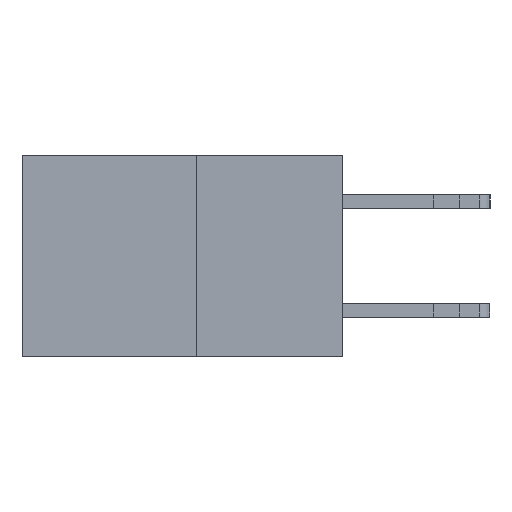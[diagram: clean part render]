
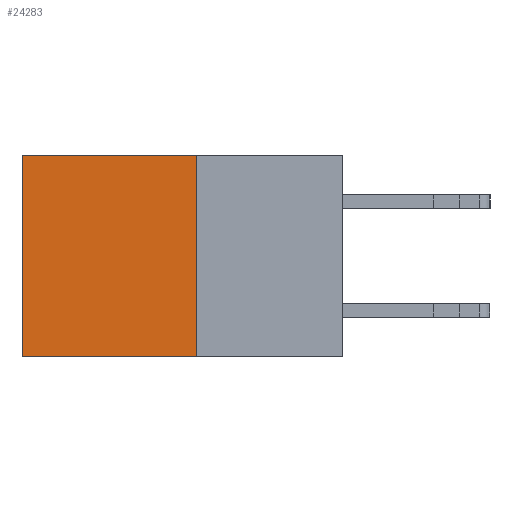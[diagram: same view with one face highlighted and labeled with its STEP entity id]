
A CAD part, left-side view. The second image highlights one B-rep face of the part: STEP entity #24283.
In plain terms, the highlighted planar face has unit normal (-1, 0, 0).
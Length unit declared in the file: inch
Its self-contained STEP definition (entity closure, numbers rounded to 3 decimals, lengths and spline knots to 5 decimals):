
#56 = DIRECTION ( 'NONE',  ( 0., 1., 0. ) ) ;
#512 = LINE ( 'NONE', #28628, #13226 ) ;
#710 = DIRECTION ( 'NONE',  ( 1., 0., 0. ) ) ;
#1823 = CARTESIAN_POINT ( 'NONE',  ( 0.277, 0.27, 0. ) ) ;
#1856 = EDGE_CURVE ( 'NONE', #9199, #30092, #512, .T. ) ;
#2623 = VECTOR ( 'NONE', #16807, 39.37008 ) ;
#3035 = CARTESIAN_POINT ( 'NONE',  ( 0.277, 0.27, -0.37 ) ) ;
#5921 = EDGE_LOOP ( 'NONE', ( #16768, #11929, #25193, #25922 ) ) ;
#8485 = VECTOR ( 'NONE', #22010, 39.37008 ) ;
#9199 = VERTEX_POINT ( 'NONE', #21758 ) ;
#9420 = VERTEX_POINT ( 'NONE', #27135 ) ;
#11929 = ORIENTED_EDGE ( 'NONE', *, *, #1856, .F. ) ;
#12901 = CARTESIAN_POINT ( 'NONE',  ( 0.277, 0.27, 0. ) ) ;
#13226 = VECTOR ( 'NONE', #56, 39.37008 ) ;
#14421 = CARTESIAN_POINT ( 'NONE',  ( 0.277, 0.59, -0.37 ) ) ;
#14996 = PLANE ( 'NONE',  #27520 ) ;
#15300 = EDGE_CURVE ( 'NONE', #21005, #9199, #18866, .T. ) ;
#16246 = FACE_OUTER_BOUND ( 'NONE', #5921, .T. ) ;
#16768 = ORIENTED_EDGE ( 'NONE', *, *, #21220, .T. ) ;
#16807 = DIRECTION ( 'NONE',  ( 0., 0., -1. ) ) ;
#16839 = VECTOR ( 'NONE', #26971, 39.37008 ) ;
#17395 = DIRECTION ( 'NONE',  ( 0., 0., -1. ) ) ;
#17869 = EDGE_CURVE ( 'NONE', #21005, #9420, #23076, .T. ) ;
#18866 = LINE ( 'NONE', #3035, #8485 ) ;
#21005 = VERTEX_POINT ( 'NONE', #1823 ) ;
#21220 = EDGE_CURVE ( 'NONE', #9420, #30092, #21556, .T. ) ;
#21556 = LINE ( 'NONE', #14421, #2623 ) ;
#21758 = CARTESIAN_POINT ( 'NONE',  ( 0.277, 0.27, -0.37 ) ) ;
#22010 = DIRECTION ( 'NONE',  ( 0., 0., -1. ) ) ;
#22809 = CARTESIAN_POINT ( 'NONE',  ( 0.277, 0.59, -0.37 ) ) ;
#23076 = LINE ( 'NONE', #12901, #16839 ) ;
#24283 = ADVANCED_FACE ( 'NONE', ( #16246 ), #14996, .F. ) ;
#25193 = ORIENTED_EDGE ( 'NONE', *, *, #15300, .F. ) ;
#25922 = ORIENTED_EDGE ( 'NONE', *, *, #17869, .T. ) ;
#26704 = CARTESIAN_POINT ( 'NONE',  ( 0.277, 0.27, -0.37 ) ) ;
#26971 = DIRECTION ( 'NONE',  ( 0., 1., 0. ) ) ;
#27135 = CARTESIAN_POINT ( 'NONE',  ( 0.277, 0.59, 0. ) ) ;
#27520 = AXIS2_PLACEMENT_3D ( 'NONE', #26704, #710, #17395 ) ;
#28628 = CARTESIAN_POINT ( 'NONE',  ( 0.277, 0.27, -0.37 ) ) ;
#30092 = VERTEX_POINT ( 'NONE', #22809 ) ;
